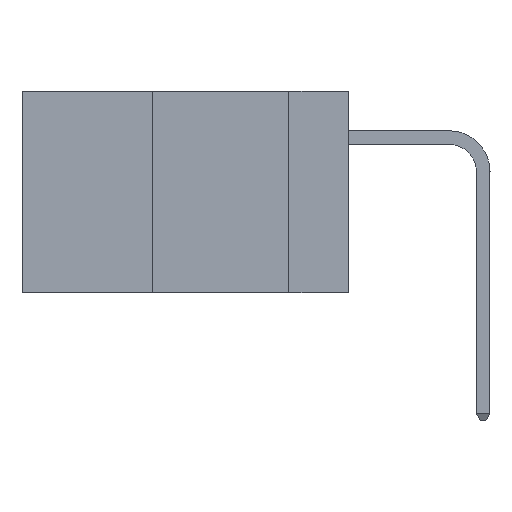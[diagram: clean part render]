
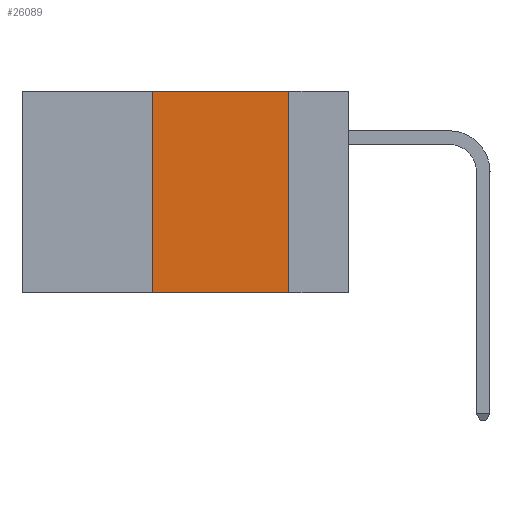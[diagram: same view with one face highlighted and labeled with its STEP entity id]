
A CAD part, left-side view. The second image highlights one B-rep face of the part: STEP entity #26089.
In plain terms, the highlighted planar face has unit normal (-1, 0, 0).
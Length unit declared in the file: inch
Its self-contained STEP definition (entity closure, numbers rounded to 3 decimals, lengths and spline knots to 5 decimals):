
#1014 = CARTESIAN_POINT ( 'NONE',  ( 0., 0.36, -0.37 ) ) ;
#1636 = CARTESIAN_POINT ( 'NONE',  ( 0., 0.36, 0. ) ) ;
#1711 = DIRECTION ( 'NONE',  ( 0., -1., 0. ) ) ;
#1893 = VECTOR ( 'NONE', #6946, 39.37008 ) ;
#2506 = EDGE_CURVE ( 'NONE', #5742, #14318, #24003, .T. ) ;
#2741 = CARTESIAN_POINT ( 'NONE',  ( 0., 0.36, 0. ) ) ;
#2783 = VERTEX_POINT ( 'NONE', #1014 ) ;
#3242 = LINE ( 'NONE', #17301, #1893 ) ;
#3481 = AXIS2_PLACEMENT_3D ( 'NONE', #24771, #12467, #26800 ) ;
#5378 = ORIENTED_EDGE ( 'NONE', *, *, #2506, .F. ) ;
#5742 = VERTEX_POINT ( 'NONE', #1636 ) ;
#6051 = CARTESIAN_POINT ( 'NONE',  ( 0., 0.6, 0. ) ) ;
#6143 = DIRECTION ( 'NONE',  ( 0., -1., 0. ) ) ;
#6946 = DIRECTION ( 'NONE',  ( 0., 0., -1. ) ) ;
#7901 = VECTOR ( 'NONE', #1711, 39.37008 ) ;
#7947 = ORIENTED_EDGE ( 'NONE', *, *, #8137, .F. ) ;
#7966 = VERTEX_POINT ( 'NONE', #20896 ) ;
#8101 = CARTESIAN_POINT ( 'NONE',  ( 0., 0.11, 0. ) ) ;
#8137 = EDGE_CURVE ( 'NONE', #14318, #7966, #3242, .T. ) ;
#9199 = DIRECTION ( 'NONE',  ( 0., 0., 1. ) ) ;
#10421 = PLANE ( 'NONE',  #3481 ) ;
#11295 = EDGE_CURVE ( 'NONE', #2783, #7966, #18852, .T. ) ;
#12467 = DIRECTION ( 'NONE',  ( 1., 0., 0. ) ) ;
#14318 = VERTEX_POINT ( 'NONE', #8101 ) ;
#15983 = VECTOR ( 'NONE', #9199, 39.37008 ) ;
#17301 = CARTESIAN_POINT ( 'NONE',  ( 0., 0.11, 0. ) ) ;
#18451 = CARTESIAN_POINT ( 'NONE',  ( 0., 0.6, -0.37 ) ) ;
#18544 = VECTOR ( 'NONE', #6143, 39.37008 ) ;
#18852 = LINE ( 'NONE', #18451, #7901 ) ;
#19178 = EDGE_CURVE ( 'NONE', #2783, #5742, #26859, .T. ) ;
#19742 = EDGE_LOOP ( 'NONE', ( #7947, #5378, #20042, #22473 ) ) ;
#20042 = ORIENTED_EDGE ( 'NONE', *, *, #19178, .F. ) ;
#20896 = CARTESIAN_POINT ( 'NONE',  ( 0., 0.11, -0.37 ) ) ;
#22164 = FACE_OUTER_BOUND ( 'NONE', #19742, .T. ) ;
#22473 = ORIENTED_EDGE ( 'NONE', *, *, #11295, .T. ) ;
#24003 = LINE ( 'NONE', #6051, #18544 ) ;
#24771 = CARTESIAN_POINT ( 'NONE',  ( 0., 0.6, 0. ) ) ;
#26089 = ADVANCED_FACE ( 'NONE', ( #22164 ), #10421, .F. ) ;
#26800 = DIRECTION ( 'NONE',  ( 0., 0., -1. ) ) ;
#26859 = LINE ( 'NONE', #2741, #15983 ) ;
